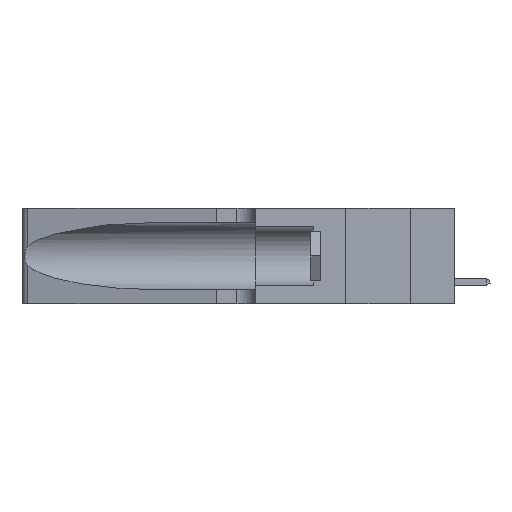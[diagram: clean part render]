
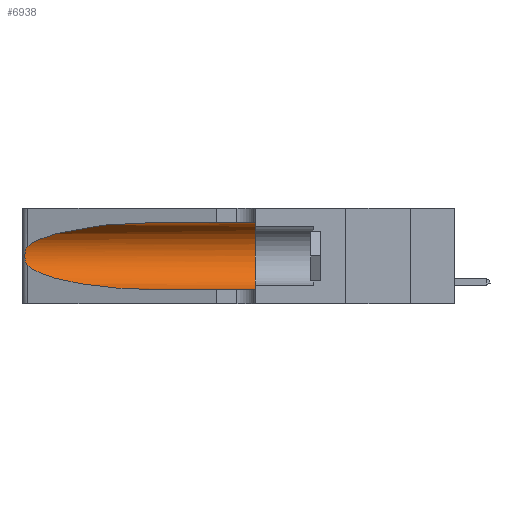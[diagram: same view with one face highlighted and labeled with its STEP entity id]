
A CAD part, left-side view. The second image highlights one B-rep face of the part: STEP entity #6938.
In plain terms, the highlighted cylindrical face has radius 3.308 mm (diameter 6.617 mm), a partial arc.
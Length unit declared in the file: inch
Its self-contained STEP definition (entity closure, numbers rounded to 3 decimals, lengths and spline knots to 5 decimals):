
#510 =( BOUNDED_CURVE ( )  B_SPLINE_CURVE ( 3, ( #3239, #29108, #33457, #30317 ),
 .UNSPECIFIED., .F., .T. ) 
 B_SPLINE_CURVE_WITH_KNOTS ( ( 4, 4 ),
 ( 1.5708, 2.84003 ),
 .UNSPECIFIED. ) 
 CURVE ( )  GEOMETRIC_REPRESENTATION_ITEM ( )  RATIONAL_B_SPLINE_CURVE ( ( 1., 0.87, 0.87, 1. ) ) 
 REPRESENTATION_ITEM ( '' )  );
#1803 = VERTEX_POINT ( 'NONE', #2293 ) ;
#2068 = CARTESIAN_POINT ( 'NONE',  ( 0.1305, 0.35, 0.185 ) ) ;
#2278 = CARTESIAN_POINT ( 'NONE',  ( 0.1305, 1.61858, 0.185 ) ) ;
#2282 = CARTESIAN_POINT ( 'NONE',  ( 0.25487, 1.22718, 0.22369 ) ) ;
#2293 = CARTESIAN_POINT ( 'NONE',  ( 0.1305, 0.35, 0.05475 ) ) ;
#2433 = CARTESIAN_POINT ( 'NONE',  ( 0.25854, 1.2359, 0.20912 ) ) ;
#2650 = VERTEX_POINT ( 'NONE', #5536 ) ;
#3239 = CARTESIAN_POINT ( 'NONE',  ( 0.1305, 0.72297, 0.31525 ) ) ;
#3948 = CARTESIAN_POINT ( 'NONE',  ( 0.25487, 1.22718, 0.14631 ) ) ;
#4895 = DIRECTION ( 'NONE',  ( 0., 0., 1. ) ) ;
#5253 = CARTESIAN_POINT ( 'NONE',  ( 0.25555, 1.22993, 0.14849 ) ) ;
#5536 = CARTESIAN_POINT ( 'NONE',  ( 0.25487, 1.22718, 0.22369 ) ) ;
#5556 = CARTESIAN_POINT ( 'NONE',  ( 0.25555, 1.22994, 0.2215 ) ) ;
#6938 = ADVANCED_FACE ( 'NONE', ( #38028 ), #28391, .F. ) ;
#7504 = CARTESIAN_POINT ( 'NONE',  ( 0.18966, 0.96281, 0.05475 ) ) ;
#7900 = CARTESIAN_POINT ( 'NONE',  ( 0.1305, 1.61858, 0.05475 ) ) ;
#8410 = AXIS2_PLACEMENT_3D ( 'NONE', #2068, #15144, #4895 ) ;
#9449 = B_SPLINE_CURVE_WITH_KNOTS ( 'NONE', 3,
 ( #2282, #5556, #31413, #30959, #2433, #15353, #28034, #37947, #21294, #18637, #24693, #25109, #5253, #14916 ),
 .UNSPECIFIED., .F., .F.,
 ( 4, 2, 2, 2, 2, 2, 4 ),
 ( 0., 0.00027, 0.00053, 0.00107, 0.0016, 0.00187, 0.00214 ),
 .UNSPECIFIED. ) ;
#9723 = DIRECTION ( 'NONE',  ( 0., -1., 0. ) ) ;
#12194 = ORIENTED_EDGE ( 'NONE', *, *, #17847, .T. ) ;
#13452 = CIRCLE ( 'NONE', #8410, 0.13025 ) ;
#14912 = DIRECTION ( 'NONE',  ( 0., 0., -1. ) ) ;
#14916 = CARTESIAN_POINT ( 'NONE',  ( 0.25487, 1.22718, 0.14631 ) ) ;
#14928 = CARTESIAN_POINT ( 'NONE',  ( 0.1305, 0.35, 0.31525 ) ) ;
#15144 = DIRECTION ( 'NONE',  ( 0., 1., 0. ) ) ;
#15353 = CARTESIAN_POINT ( 'NONE',  ( 0.26018, 1.23835, 0.19895 ) ) ;
#17847 = EDGE_CURVE ( 'NONE', #23124, #2650, #510, .T. ) ;
#18573 = EDGE_CURVE ( 'NONE', #2650, #33641, #9449, .T. ) ;
#18637 = CARTESIAN_POINT ( 'NONE',  ( 0.25856, 1.23593, 0.16098 ) ) ;
#19662 = ORIENTED_EDGE ( 'NONE', *, *, #18573, .T. ) ;
#20936 = ORIENTED_EDGE ( 'NONE', *, *, #27170, .T. ) ;
#21294 = CARTESIAN_POINT ( 'NONE',  ( 0.26017, 1.23833, 0.17102 ) ) ;
#21361 =( BOUNDED_CURVE ( )  B_SPLINE_CURVE ( 3, ( #3948, #26619, #7504, #30100 ),
 .UNSPECIFIED., .F., .F. ) 
 B_SPLINE_CURVE_WITH_KNOTS ( ( 4, 4 ),
 ( 3.44316, 4.71239 ),
 .UNSPECIFIED. ) 
 CURVE ( )  GEOMETRIC_REPRESENTATION_ITEM ( )  RATIONAL_B_SPLINE_CURVE ( ( 1., 0.87, 0.87, 1. ) ) 
 REPRESENTATION_ITEM ( '' )  );
#21611 = EDGE_CURVE ( 'NONE', #37552, #1803, #13452, .T. ) ;
#23124 = VERTEX_POINT ( 'NONE', #30258 ) ;
#24693 = CARTESIAN_POINT ( 'NONE',  ( 0.25789, 1.23486, 0.15765 ) ) ;
#25109 = CARTESIAN_POINT ( 'NONE',  ( 0.25639, 1.23186, 0.15144 ) ) ;
#25391 = VECTOR ( 'NONE', #9723, 39.37008 ) ;
#25437 = CARTESIAN_POINT ( 'NONE',  ( 0.1305, 1.61858, 0.31525 ) ) ;
#26619 = CARTESIAN_POINT ( 'NONE',  ( 0.2373, 1.15595, 0.08982 ) ) ;
#27170 = EDGE_CURVE ( 'NONE', #33641, #36779, #21361, .T. ) ;
#28030 = DIRECTION ( 'NONE',  ( 0., -1., 0. ) ) ;
#28034 = CARTESIAN_POINT ( 'NONE',  ( 0.26075, 1.23896, 0.19203 ) ) ;
#28391 = CYLINDRICAL_SURFACE ( 'NONE', #38881, 0.13025 ) ;
#28549 = EDGE_LOOP ( 'NONE', ( #12194, #19662, #20936, #35708, #38416, #34562 ) ) ;
#29108 = CARTESIAN_POINT ( 'NONE',  ( 0.18966, 0.96281, 0.31525 ) ) ;
#29662 = EDGE_CURVE ( 'NONE', #36779, #1803, #29763, .T. ) ;
#29763 = LINE ( 'NONE', #7900, #36914 ) ;
#30100 = CARTESIAN_POINT ( 'NONE',  ( 0.1305, 0.72297, 0.05475 ) ) ;
#30258 = CARTESIAN_POINT ( 'NONE',  ( 0.1305, 0.72297, 0.31525 ) ) ;
#30317 = CARTESIAN_POINT ( 'NONE',  ( 0.25487, 1.22718, 0.22369 ) ) ;
#30959 = CARTESIAN_POINT ( 'NONE',  ( 0.25787, 1.23484, 0.2124 ) ) ;
#31413 = CARTESIAN_POINT ( 'NONE',  ( 0.25639, 1.23184, 0.21858 ) ) ;
#32778 = CARTESIAN_POINT ( 'NONE',  ( 0.1305, 0.72297, 0.05475 ) ) ;
#33457 = CARTESIAN_POINT ( 'NONE',  ( 0.2373, 1.15595, 0.28018 ) ) ;
#33522 = CARTESIAN_POINT ( 'NONE',  ( 0.25487, 1.22718, 0.14631 ) ) ;
#33641 = VERTEX_POINT ( 'NONE', #33522 ) ;
#33929 = LINE ( 'NONE', #25437, #25391 ) ;
#34562 = ORIENTED_EDGE ( 'NONE', *, *, #35151, .F. ) ;
#35151 = EDGE_CURVE ( 'NONE', #23124, #37552, #33929, .T. ) ;
#35708 = ORIENTED_EDGE ( 'NONE', *, *, #29662, .T. ) ;
#36779 = VERTEX_POINT ( 'NONE', #32778 ) ;
#36914 = VECTOR ( 'NONE', #37177, 39.37008 ) ;
#37177 = DIRECTION ( 'NONE',  ( 0., -1., 0. ) ) ;
#37552 = VERTEX_POINT ( 'NONE', #14928 ) ;
#37947 = CARTESIAN_POINT ( 'NONE',  ( 0.26075, 1.23896, 0.178 ) ) ;
#38028 = FACE_OUTER_BOUND ( 'NONE', #28549, .T. ) ;
#38416 = ORIENTED_EDGE ( 'NONE', *, *, #21611, .F. ) ;
#38881 = AXIS2_PLACEMENT_3D ( 'NONE', #2278, #28030, #14912 ) ;
